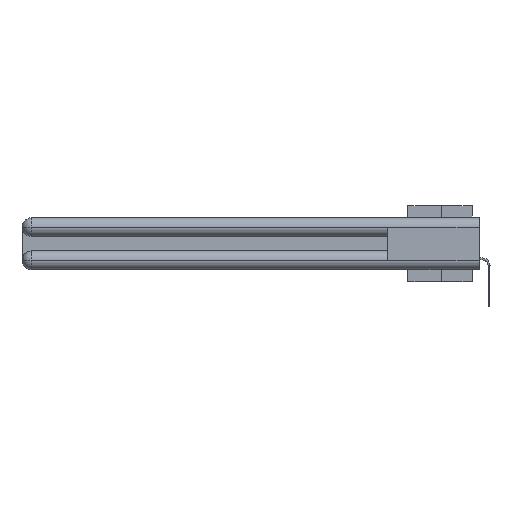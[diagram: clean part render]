
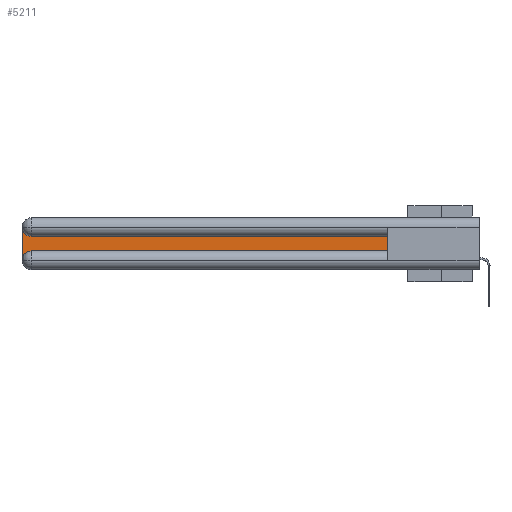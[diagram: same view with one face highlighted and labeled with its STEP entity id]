
A CAD part, left-side view. The second image highlights one B-rep face of the part: STEP entity #5211.
In plain terms, the highlighted planar face has unit normal (-1, 0, 0).
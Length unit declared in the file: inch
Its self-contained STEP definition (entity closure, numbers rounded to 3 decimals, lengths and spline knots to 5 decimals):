
#160 = CARTESIAN_POINT ( 'NONE',  ( 0.075, 3., -0.2775 ) ) ;
#873 = EDGE_CURVE ( 'NONE', #8942, #6080, #24943, .T. ) ;
#1272 = EDGE_CURVE ( 'NONE', #26381, #8942, #14352, .T. ) ;
#1509 = DIRECTION ( 'NONE',  ( 0., 1., 0. ) ) ;
#2337 = CARTESIAN_POINT ( 'NONE',  ( 0.075, 3., -0.0625 ) ) ;
#2457 = AXIS2_PLACEMENT_3D ( 'NONE', #16552, #19341, #11576 ) ;
#2870 = ORIENTED_EDGE ( 'NONE', *, *, #24233, .T. ) ;
#4740 = CARTESIAN_POINT ( 'NONE',  ( 0.075, 2.94, -0.1225 ) ) ;
#5211 = ADVANCED_FACE ( 'NONE', ( #23486 ), #30467, .F. ) ;
#6031 = CARTESIAN_POINT ( 'NONE',  ( 0.075, 2.94, -0.2175 ) ) ;
#6080 = VERTEX_POINT ( 'NONE', #4740 ) ;
#6273 = ORIENTED_EDGE ( 'NONE', *, *, #30613, .T. ) ;
#6483 = CIRCLE ( 'NONE', #10940, 0.06 ) ;
#7453 = CARTESIAN_POINT ( 'NONE',  ( 0.075, 3., -0.2175 ) ) ;
#7760 = LINE ( 'NONE', #7453, #12148 ) ;
#8330 = VERTEX_POINT ( 'NONE', #160 ) ;
#8942 = VERTEX_POINT ( 'NONE', #28619 ) ;
#9902 = CARTESIAN_POINT ( 'NONE',  ( 0.075, 0.6, -0.2175 ) ) ;
#10626 = DIRECTION ( 'NONE',  ( 0., 0., 1. ) ) ;
#10940 = AXIS2_PLACEMENT_3D ( 'NONE', #28433, #11818, #21466 ) ;
#11576 = DIRECTION ( 'NONE',  ( 0., 0., -1. ) ) ;
#11818 = DIRECTION ( 'NONE',  ( 1., 0., 0. ) ) ;
#12148 = VECTOR ( 'NONE', #12418, 39.37008 ) ;
#12418 = DIRECTION ( 'NONE',  ( 0., 0., -1. ) ) ;
#13709 = DIRECTION ( 'NONE',  ( 0., 0., -1. ) ) ;
#14352 = LINE ( 'NONE', #17611, #27487 ) ;
#16543 = AXIS2_PLACEMENT_3D ( 'NONE', #21320, #18980, #13709 ) ;
#16552 = CARTESIAN_POINT ( 'NONE',  ( 0.075, 2.94, -0.0625 ) ) ;
#16740 = EDGE_CURVE ( 'NONE', #8330, #17465, #6483, .T. ) ;
#17465 = VERTEX_POINT ( 'NONE', #6031 ) ;
#17504 = ORIENTED_EDGE ( 'NONE', *, *, #16740, .T. ) ;
#17611 = CARTESIAN_POINT ( 'NONE',  ( 0.075, 0.6, -0.2175 ) ) ;
#17787 = CIRCLE ( 'NONE', #2457, 0.06 ) ;
#18980 = DIRECTION ( 'NONE',  ( 1., 0., 0. ) ) ;
#19207 = ORIENTED_EDGE ( 'NONE', *, *, #1272, .T. ) ;
#19341 = DIRECTION ( 'NONE',  ( 1., 0., 0. ) ) ;
#20737 = CARTESIAN_POINT ( 'NONE',  ( 0.075, 0.6, -0.2175 ) ) ;
#21320 = CARTESIAN_POINT ( 'NONE',  ( 0.075, 3., -0.1225 ) ) ;
#21466 = DIRECTION ( 'NONE',  ( 0., 0., -1. ) ) ;
#21713 = LINE ( 'NONE', #9902, #28008 ) ;
#22517 = VECTOR ( 'NONE', #1509, 39.37008 ) ;
#23026 = VERTEX_POINT ( 'NONE', #2337 ) ;
#23437 = EDGE_CURVE ( 'NONE', #17465, #26381, #21713, .T. ) ;
#23486 = FACE_OUTER_BOUND ( 'NONE', #25745, .T. ) ;
#24233 = EDGE_CURVE ( 'NONE', #23026, #8330, #7760, .T. ) ;
#24641 = CARTESIAN_POINT ( 'NONE',  ( 0.075, 0.6, -0.1225 ) ) ;
#24806 = ORIENTED_EDGE ( 'NONE', *, *, #873, .T. ) ;
#24943 = LINE ( 'NONE', #24641, #22517 ) ;
#25745 = EDGE_LOOP ( 'NONE', ( #24806, #6273, #2870, #17504, #29892, #19207 ) ) ;
#26381 = VERTEX_POINT ( 'NONE', #20737 ) ;
#27487 = VECTOR ( 'NONE', #10626, 39.37008 ) ;
#28008 = VECTOR ( 'NONE', #28521, 39.37008 ) ;
#28433 = CARTESIAN_POINT ( 'NONE',  ( 0.075, 2.94, -0.2775 ) ) ;
#28521 = DIRECTION ( 'NONE',  ( 0., -1., 0. ) ) ;
#28619 = CARTESIAN_POINT ( 'NONE',  ( 0.075, 0.6, -0.1225 ) ) ;
#29892 = ORIENTED_EDGE ( 'NONE', *, *, #23437, .T. ) ;
#30467 = PLANE ( 'NONE',  #16543 ) ;
#30613 = EDGE_CURVE ( 'NONE', #6080, #23026, #17787, .T. ) ;
